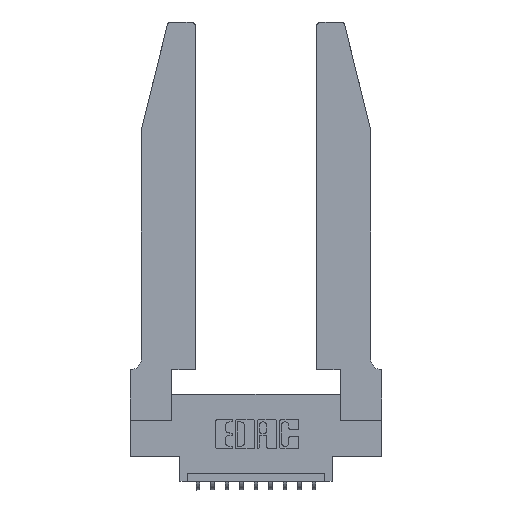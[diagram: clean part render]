
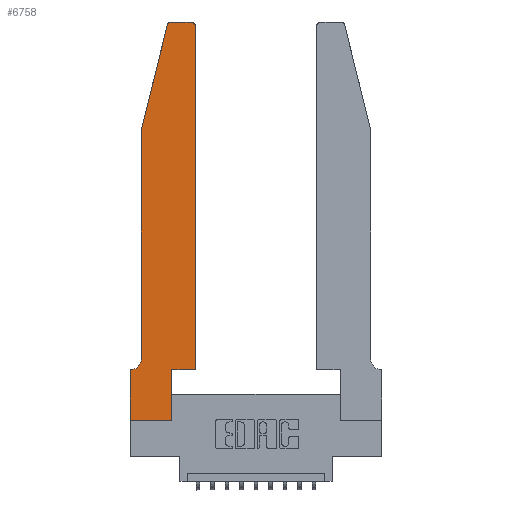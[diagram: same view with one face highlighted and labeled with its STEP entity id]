
A CAD part, top view. The second image highlights one B-rep face of the part: STEP entity #6758.
In plain terms, the highlighted planar face has unit normal (0, 0, 1).
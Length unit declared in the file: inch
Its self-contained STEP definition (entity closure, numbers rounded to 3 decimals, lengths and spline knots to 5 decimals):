
#226 = VECTOR ( 'NONE', #10580, 39.37008 ) ;
#241 = LINE ( 'NONE', #4440, #15071 ) ;
#276 = EDGE_CURVE ( 'NONE', #13418, #2355, #13509, .T. ) ;
#296 = CARTESIAN_POINT ( 'NONE',  ( 0.4205, 2.72, 0.37 ) ) ;
#561 = ORIENTED_EDGE ( 'NONE', *, *, #3875, .T. ) ;
#694 = AXIS2_PLACEMENT_3D ( 'NONE', #14736, #16068, #7259 ) ;
#969 = CARTESIAN_POINT ( 'NONE',  ( 0.2865, 0., 0.37 ) ) ;
#1060 = ORIENTED_EDGE ( 'NONE', *, *, #14375, .T. ) ;
#1061 = EDGE_CURVE ( 'NONE', #8424, #14701, #4690, .T. ) ;
#1078 = ORIENTED_EDGE ( 'NONE', *, *, #1141, .T. ) ;
#1141 = EDGE_CURVE ( 'NONE', #11136, #5157, #3116, .T. ) ;
#1208 = LINE ( 'NONE', #7730, #11755 ) ;
#1211 = CARTESIAN_POINT ( 'NONE',  ( 0.284, 2.75, 0.37 ) ) ;
#1231 = DIRECTION ( 'NONE',  ( 0., 0., 1. ) ) ;
#1433 = ORIENTED_EDGE ( 'NONE', *, *, #14007, .T. ) ;
#1952 = VECTOR ( 'NONE', #10224, 39.37008 ) ;
#1977 = DIRECTION ( 'NONE',  ( -1., 0., 0. ) ) ;
#2337 = EDGE_LOOP ( 'NONE', ( #561, #6516, #12155, #1060, #13781, #1433, #13240, #12500, #1078, #10541, #6315, #15948 ) ) ;
#2355 = VERTEX_POINT ( 'NONE', #14876 ) ;
#2365 = CARTESIAN_POINT ( 'NONE',  ( 0.2605, 2.75, 0.37 ) ) ;
#2702 = CARTESIAN_POINT ( 'NONE',  ( 0., 0., 0.37 ) ) ;
#2773 = CIRCLE ( 'NONE', #4892, 0.03 ) ;
#3116 = LINE ( 'NONE', #3494, #9137 ) ;
#3482 = DIRECTION ( 'NONE',  ( -1., 0., 0. ) ) ;
#3494 = CARTESIAN_POINT ( 'NONE',  ( 0.2865, 0.35, 0.37 ) ) ;
#3727 = VECTOR ( 'NONE', #8078, 39.37008 ) ;
#3875 = EDGE_CURVE ( 'NONE', #14102, #8424, #8786, .T. ) ;
#3940 = DIRECTION ( 'NONE',  ( 1., 0., 0. ) ) ;
#4321 = AXIS2_PLACEMENT_3D ( 'NONE', #7537, #1231, #3940 ) ;
#4440 = CARTESIAN_POINT ( 'NONE',  ( 0.0755, 0.35, 0.37 ) ) ;
#4476 = VERTEX_POINT ( 'NONE', #6206 ) ;
#4548 = EDGE_CURVE ( 'NONE', #4476, #6391, #6086, .T. ) ;
#4690 = CIRCLE ( 'NONE', #7358, 0.03 ) ;
#4892 = AXIS2_PLACEMENT_3D ( 'NONE', #296, #7869, #14110 ) ;
#5157 = VERTEX_POINT ( 'NONE', #5376 ) ;
#5376 = CARTESIAN_POINT ( 'NONE',  ( 0.2865, 0.35, 0.37 ) ) ;
#5529 = DIRECTION ( 'NONE',  ( 0., 1., 0. ) ) ;
#5547 = DIRECTION ( 'NONE',  ( 0., 0., 1. ) ) ;
#5582 = EDGE_CURVE ( 'NONE', #5157, #13418, #11116, .T. ) ;
#5618 = CARTESIAN_POINT ( 'NONE',  ( 0., 0., 0.37 ) ) ;
#5670 = LINE ( 'NONE', #2702, #1952 ) ;
#5887 = VECTOR ( 'NONE', #5529, 39.37008 ) ;
#6086 = CIRCLE ( 'NONE', #694, 0.07 ) ;
#6206 = CARTESIAN_POINT ( 'NONE',  ( 0.0755, 0.42, 0.37 ) ) ;
#6315 = ORIENTED_EDGE ( 'NONE', *, *, #276, .T. ) ;
#6391 = VERTEX_POINT ( 'NONE', #15556 ) ;
#6516 = ORIENTED_EDGE ( 'NONE', *, *, #1061, .T. ) ;
#6758 = ADVANCED_FACE ( 'NONE', ( #12224 ), #14972, .T. ) ;
#7259 = DIRECTION ( 'NONE',  ( -1., 0., 0. ) ) ;
#7358 = AXIS2_PLACEMENT_3D ( 'NONE', #15757, #5547, #8029 ) ;
#7537 = CARTESIAN_POINT ( 'NONE',  ( 0., 0.35, 0.37 ) ) ;
#7628 = CARTESIAN_POINT ( 'NONE',  ( 0.4505, 0.35, 0.37 ) ) ;
#7730 = CARTESIAN_POINT ( 'NONE',  ( 0.0755, 2., 0.37 ) ) ;
#7756 = CARTESIAN_POINT ( 'NONE',  ( 0.4505, 0.35, 0.37 ) ) ;
#7869 = DIRECTION ( 'NONE',  ( 0., 0., 1. ) ) ;
#8029 = DIRECTION ( 'NONE',  ( 1., 0., 0. ) ) ;
#8078 = DIRECTION ( 'NONE',  ( -0.239, -0.971, 0. ) ) ;
#8424 = VERTEX_POINT ( 'NONE', #1211 ) ;
#8497 = CARTESIAN_POINT ( 'NONE',  ( 0.4205, 2.75, 0.37 ) ) ;
#8786 = LINE ( 'NONE', #2365, #15061 ) ;
#8959 = DIRECTION ( 'NONE',  ( 1., 0., 0. ) ) ;
#9048 = EDGE_CURVE ( 'NONE', #12110, #11136, #5670, .T. ) ;
#9137 = VECTOR ( 'NONE', #10830, 39.37008 ) ;
#9195 = CARTESIAN_POINT ( 'NONE',  ( 0., 0., 0.37 ) ) ;
#9742 = EDGE_CURVE ( 'NONE', #14701, #15216, #13665, .T. ) ;
#10224 = DIRECTION ( 'NONE',  ( 1., 0., 0. ) ) ;
#10541 = ORIENTED_EDGE ( 'NONE', *, *, #5582, .T. ) ;
#10580 = DIRECTION ( 'NONE',  ( 0., -1., 0. ) ) ;
#10679 = CARTESIAN_POINT ( 'NONE',  ( 0., 0.35, 0.37 ) ) ;
#10830 = DIRECTION ( 'NONE',  ( 0., 1., 0. ) ) ;
#11116 = LINE ( 'NONE', #7756, #13848 ) ;
#11136 = VERTEX_POINT ( 'NONE', #969 ) ;
#11524 = DIRECTION ( 'NONE',  ( 0., -1., 0. ) ) ;
#11755 = VECTOR ( 'NONE', #11524, 39.37008 ) ;
#11815 = CARTESIAN_POINT ( 'NONE',  ( 0.0755, 2., 0.37 ) ) ;
#12110 = VERTEX_POINT ( 'NONE', #9195 ) ;
#12155 = ORIENTED_EDGE ( 'NONE', *, *, #9742, .T. ) ;
#12224 = FACE_OUTER_BOUND ( 'NONE', #2337, .T. ) ;
#12500 = ORIENTED_EDGE ( 'NONE', *, *, #9048, .T. ) ;
#12803 = VERTEX_POINT ( 'NONE', #10679 ) ;
#13240 = ORIENTED_EDGE ( 'NONE', *, *, #14456, .T. ) ;
#13418 = VERTEX_POINT ( 'NONE', #14369 ) ;
#13509 = LINE ( 'NONE', #7628, #5887 ) ;
#13533 = LINE ( 'NONE', #5618, #226 ) ;
#13665 = LINE ( 'NONE', #11815, #3727 ) ;
#13781 = ORIENTED_EDGE ( 'NONE', *, *, #4548, .T. ) ;
#13848 = VECTOR ( 'NONE', #8959, 39.37008 ) ;
#14007 = EDGE_CURVE ( 'NONE', #6391, #12803, #241, .T. ) ;
#14102 = VERTEX_POINT ( 'NONE', #8497 ) ;
#14110 = DIRECTION ( 'NONE',  ( 1., 0., 0. ) ) ;
#14369 = CARTESIAN_POINT ( 'NONE',  ( 0.4505, 0.35, 0.37 ) ) ;
#14375 = EDGE_CURVE ( 'NONE', #15216, #4476, #1208, .T. ) ;
#14456 = EDGE_CURVE ( 'NONE', #12803, #12110, #13533, .T. ) ;
#14701 = VERTEX_POINT ( 'NONE', #14925 ) ;
#14736 = CARTESIAN_POINT ( 'NONE',  ( 0.0055, 0.42, 0.37 ) ) ;
#14876 = CARTESIAN_POINT ( 'NONE',  ( 0.4505, 2.72, 0.37 ) ) ;
#14925 = CARTESIAN_POINT ( 'NONE',  ( 0.25487, 2.72718, 0.37 ) ) ;
#14972 = PLANE ( 'NONE',  #4321 ) ;
#14999 = EDGE_CURVE ( 'NONE', #2355, #14102, #2773, .T. ) ;
#15061 = VECTOR ( 'NONE', #3482, 39.37008 ) ;
#15071 = VECTOR ( 'NONE', #1977, 39.37008 ) ;
#15216 = VERTEX_POINT ( 'NONE', #15521 ) ;
#15521 = CARTESIAN_POINT ( 'NONE',  ( 0.0755, 2., 0.37 ) ) ;
#15556 = CARTESIAN_POINT ( 'NONE',  ( 0.0055, 0.35, 0.37 ) ) ;
#15757 = CARTESIAN_POINT ( 'NONE',  ( 0.284, 2.72, 0.37 ) ) ;
#15948 = ORIENTED_EDGE ( 'NONE', *, *, #14999, .T. ) ;
#16068 = DIRECTION ( 'NONE',  ( 0., 0., -1. ) ) ;
